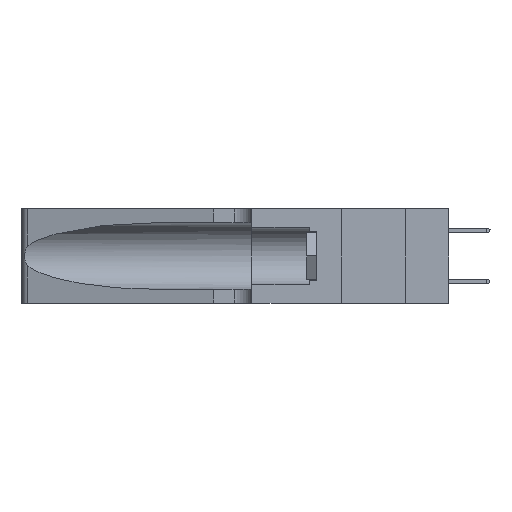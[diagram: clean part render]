
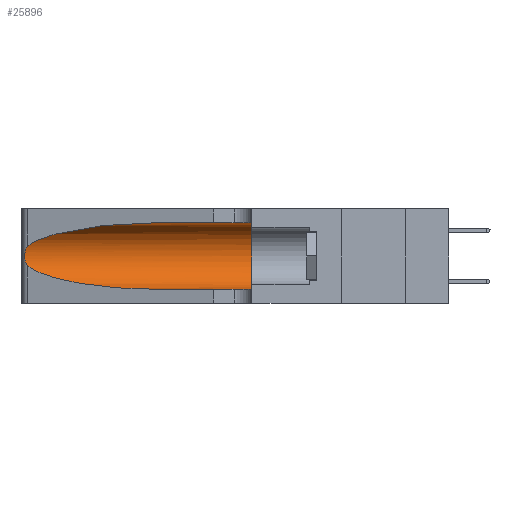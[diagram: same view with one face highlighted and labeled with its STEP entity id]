
A CAD part, left-side view. The second image highlights one B-rep face of the part: STEP entity #25896.
In plain terms, the highlighted cylindrical face has radius 3.308 mm (diameter 6.617 mm), a partial arc.
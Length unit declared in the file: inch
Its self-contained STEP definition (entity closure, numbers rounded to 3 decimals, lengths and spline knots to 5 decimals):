
#90 = VERTEX_POINT ( 'NONE', #900 ) ;
#900 = CARTESIAN_POINT ( 'NONE',  ( 0.1305, 0.72297, 0.05475 ) ) ;
#1779 = EDGE_CURVE ( 'NONE', #36563, #90, #3722, .T. ) ;
#1990 = CARTESIAN_POINT ( 'NONE',  ( 0.1305, 0.72297, 0.31525 ) ) ;
#2042 = CARTESIAN_POINT ( 'NONE',  ( 0.25854, 1.2359, 0.20912 ) ) ;
#2533 = CARTESIAN_POINT ( 'NONE',  ( 0.25487, 1.22718, 0.14631 ) ) ;
#3038 = AXIS2_PLACEMENT_3D ( 'NONE', #33564, #14811, #36668 ) ;
#3214 = CARTESIAN_POINT ( 'NONE',  ( 0.25487, 1.22718, 0.22369 ) ) ;
#3722 =( BOUNDED_CURVE ( )  B_SPLINE_CURVE ( 3, ( #2533, #15050, #5717, #27656 ),
 .UNSPECIFIED., .F., .F. ) 
 B_SPLINE_CURVE_WITH_KNOTS ( ( 4, 4 ),
 ( 3.44316, 4.71239 ),
 .UNSPECIFIED. ) 
 CURVE ( )  GEOMETRIC_REPRESENTATION_ITEM ( )  RATIONAL_B_SPLINE_CURVE ( ( 1., 0.87, 0.87, 1. ) ) 
 REPRESENTATION_ITEM ( '' )  );
#4021 = CYLINDRICAL_SURFACE ( 'NONE', #29353, 0.13025 ) ;
#4987 = ORIENTED_EDGE ( 'NONE', *, *, #13564, .T. ) ;
#5118 = ORIENTED_EDGE ( 'NONE', *, *, #12855, .T. ) ;
#5215 = CARTESIAN_POINT ( 'NONE',  ( 0.26075, 1.23896, 0.19203 ) ) ;
#5384 = VECTOR ( 'NONE', #21135, 39.37008 ) ;
#5717 = CARTESIAN_POINT ( 'NONE',  ( 0.18966, 0.96281, 0.05475 ) ) ;
#7393 = ORIENTED_EDGE ( 'NONE', *, *, #29773, .F. ) ;
#8417 = CARTESIAN_POINT ( 'NONE',  ( 0.26017, 1.23833, 0.17102 ) ) ;
#9621 = CIRCLE ( 'NONE', #3038, 0.13025 ) ;
#11574 = CARTESIAN_POINT ( 'NONE',  ( 0.25789, 1.23486, 0.15765 ) ) ;
#11890 = VERTEX_POINT ( 'NONE', #13556 ) ;
#12855 = EDGE_CURVE ( 'NONE', #90, #11890, #32379, .T. ) ;
#13556 = CARTESIAN_POINT ( 'NONE',  ( 0.1305, 0.35, 0.05475 ) ) ;
#13564 = EDGE_CURVE ( 'NONE', #28695, #36563, #15303, .T. ) ;
#14398 = DIRECTION ( 'NONE',  ( 0., -1., 0. ) ) ;
#14582 = CARTESIAN_POINT ( 'NONE',  ( 0.25487, 1.22718, 0.22369 ) ) ;
#14718 = CARTESIAN_POINT ( 'NONE',  ( 0.25555, 1.22993, 0.14849 ) ) ;
#14811 = DIRECTION ( 'NONE',  ( 0., 1., 0. ) ) ;
#15050 = CARTESIAN_POINT ( 'NONE',  ( 0.2373, 1.15595, 0.08982 ) ) ;
#15303 = B_SPLINE_CURVE_WITH_KNOTS ( 'NONE', 3,
 ( #14582, #17720, #39532, #20865, #2042, #24009, #5215, #27166, #8417, #30321, #11574, #33466, #14718, #36575 ),
 .UNSPECIFIED., .F., .F.,
 ( 4, 2, 2, 2, 2, 2, 4 ),
 ( 0., 0.00027, 0.00053, 0.00107, 0.0016, 0.00187, 0.00214 ),
 .UNSPECIFIED. ) ;
#16276 = CARTESIAN_POINT ( 'NONE',  ( 0.1305, 1.61858, 0.31525 ) ) ;
#16993 = VERTEX_POINT ( 'NONE', #1990 ) ;
#17720 = CARTESIAN_POINT ( 'NONE',  ( 0.25555, 1.22994, 0.2215 ) ) ;
#19421 = DIRECTION ( 'NONE',  ( 0., -1., 0. ) ) ;
#19544 = EDGE_CURVE ( 'NONE', #16993, #28695, #34126, .T. ) ;
#20441 = LINE ( 'NONE', #16276, #36101 ) ;
#20584 = ORIENTED_EDGE ( 'NONE', *, *, #24278, .F. ) ;
#20865 = CARTESIAN_POINT ( 'NONE',  ( 0.25787, 1.23484, 0.2124 ) ) ;
#20993 = CARTESIAN_POINT ( 'NONE',  ( 0.1305, 1.61858, 0.05475 ) ) ;
#21135 = DIRECTION ( 'NONE',  ( 0., -1., 0. ) ) ;
#22022 = CARTESIAN_POINT ( 'NONE',  ( 0.2373, 1.15595, 0.28018 ) ) ;
#23309 = CARTESIAN_POINT ( 'NONE',  ( 0.25487, 1.22718, 0.14631 ) ) ;
#24009 = CARTESIAN_POINT ( 'NONE',  ( 0.26018, 1.23835, 0.19895 ) ) ;
#24278 = EDGE_CURVE ( 'NONE', #32372, #11890, #9621, .T. ) ;
#25362 = EDGE_LOOP ( 'NONE', ( #35908, #4987, #30709, #5118, #20584, #7393 ) ) ;
#25896 = ADVANCED_FACE ( 'NONE', ( #38299 ), #4021, .F. ) ;
#27166 = CARTESIAN_POINT ( 'NONE',  ( 0.26075, 1.23896, 0.178 ) ) ;
#27656 = CARTESIAN_POINT ( 'NONE',  ( 0.1305, 0.72297, 0.05475 ) ) ;
#28695 = VERTEX_POINT ( 'NONE', #29226 ) ;
#29226 = CARTESIAN_POINT ( 'NONE',  ( 0.25487, 1.22718, 0.22369 ) ) ;
#29353 = AXIS2_PLACEMENT_3D ( 'NONE', #29986, #14398, #36254 ) ;
#29773 = EDGE_CURVE ( 'NONE', #16993, #32372, #20441, .T. ) ;
#29986 = CARTESIAN_POINT ( 'NONE',  ( 0.1305, 1.61858, 0.185 ) ) ;
#30321 = CARTESIAN_POINT ( 'NONE',  ( 0.25856, 1.23593, 0.16098 ) ) ;
#30709 = ORIENTED_EDGE ( 'NONE', *, *, #1779, .T. ) ;
#32372 = VERTEX_POINT ( 'NONE', #33850 ) ;
#32379 = LINE ( 'NONE', #20993, #5384 ) ;
#33466 = CARTESIAN_POINT ( 'NONE',  ( 0.25639, 1.23186, 0.15144 ) ) ;
#33564 = CARTESIAN_POINT ( 'NONE',  ( 0.1305, 0.35, 0.185 ) ) ;
#33850 = CARTESIAN_POINT ( 'NONE',  ( 0.1305, 0.35, 0.31525 ) ) ;
#34126 =( BOUNDED_CURVE ( )  B_SPLINE_CURVE ( 3, ( #34461, #37570, #22022, #3214 ),
 .UNSPECIFIED., .F., .T. ) 
 B_SPLINE_CURVE_WITH_KNOTS ( ( 4, 4 ),
 ( 1.5708, 2.84003 ),
 .UNSPECIFIED. ) 
 CURVE ( )  GEOMETRIC_REPRESENTATION_ITEM ( )  RATIONAL_B_SPLINE_CURVE ( ( 1., 0.87, 0.87, 1. ) ) 
 REPRESENTATION_ITEM ( '' )  );
#34461 = CARTESIAN_POINT ( 'NONE',  ( 0.1305, 0.72297, 0.31525 ) ) ;
#35908 = ORIENTED_EDGE ( 'NONE', *, *, #19544, .T. ) ;
#36101 = VECTOR ( 'NONE', #19421, 39.37008 ) ;
#36254 = DIRECTION ( 'NONE',  ( 0., 0., -1. ) ) ;
#36563 = VERTEX_POINT ( 'NONE', #23309 ) ;
#36575 = CARTESIAN_POINT ( 'NONE',  ( 0.25487, 1.22718, 0.14631 ) ) ;
#36668 = DIRECTION ( 'NONE',  ( 0., 0., 1. ) ) ;
#37570 = CARTESIAN_POINT ( 'NONE',  ( 0.18966, 0.96281, 0.31525 ) ) ;
#38299 = FACE_OUTER_BOUND ( 'NONE', #25362, .T. ) ;
#39532 = CARTESIAN_POINT ( 'NONE',  ( 0.25639, 1.23184, 0.21858 ) ) ;
